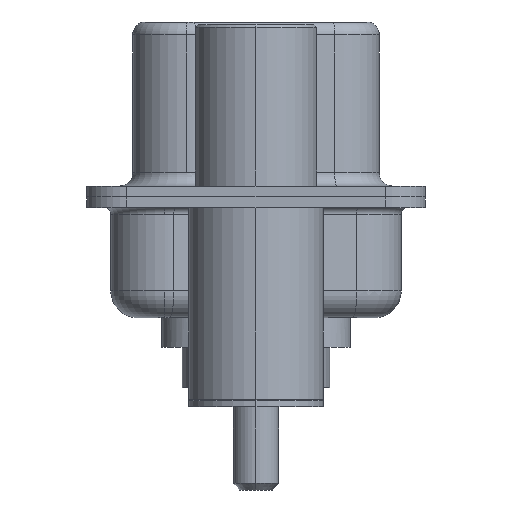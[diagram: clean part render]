
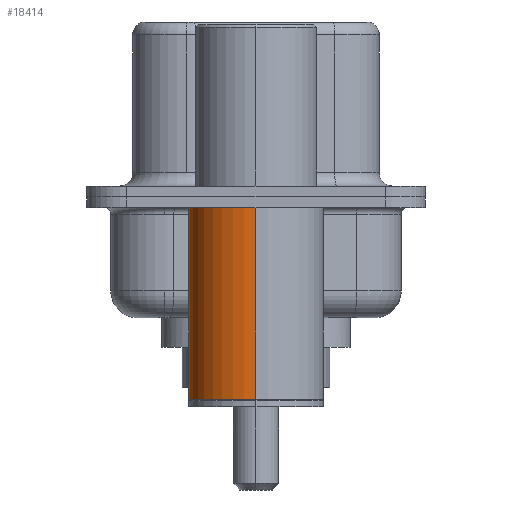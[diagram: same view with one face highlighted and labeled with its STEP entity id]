
A CAD part, left-side view. The second image highlights one B-rep face of the part: STEP entity #18414.
In plain terms, the highlighted cylindrical face has radius 2.5 mm (diameter 5 mm), a partial arc.
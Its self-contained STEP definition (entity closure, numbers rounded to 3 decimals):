
#73 = VERTEX_POINT ( 'NONE', #21918 ) ;
#85 = ORIENTED_EDGE ( 'NONE', *, *, #19931, .T. ) ;
#529 = AXIS2_PLACEMENT_3D ( 'NONE', #9377, #18113, #21693 ) ;
#629 = ORIENTED_EDGE ( 'NONE', *, *, #5912, .F. ) ;
#871 = DIRECTION ( 'NONE',  ( 0., 0., 1. ) ) ;
#2914 = AXIS2_PLACEMENT_3D ( 'NONE', #13565, #18000, #12111 ) ;
#3338 = VERTEX_POINT ( 'NONE', #3787 ) ;
#3787 = CARTESIAN_POINT ( 'NONE',  ( -2.5, 0., -0.4 ) ) ;
#4236 = FACE_OUTER_BOUND ( 'NONE', #6891, .T. ) ;
#5479 = DIRECTION ( 'NONE',  ( 0., 0., 1. ) ) ;
#5726 = CARTESIAN_POINT ( 'NONE',  ( 0., 0., -7.525 ) ) ;
#5912 = EDGE_CURVE ( 'NONE', #7821, #3338, #6349, .T. ) ;
#5987 = CARTESIAN_POINT ( 'NONE',  ( 2.5, 0., -0.4 ) ) ;
#6349 = CIRCLE ( 'NONE', #2914, 2.5 ) ;
#6891 = EDGE_LOOP ( 'NONE', ( #17485, #85, #629, #15341 ) ) ;
#7402 = DIRECTION ( 'NONE',  ( 1., 0., 0. ) ) ;
#7821 = VERTEX_POINT ( 'NONE', #5987 ) ;
#8717 = LINE ( 'NONE', #8789, #17523 ) ;
#8789 = CARTESIAN_POINT ( 'NONE',  ( -2.5, 0., 0.581 ) ) ;
#9377 = CARTESIAN_POINT ( 'NONE',  ( 0., 0., 0.581 ) ) ;
#12032 = LINE ( 'NONE', #21799, #15036 ) ;
#12111 = DIRECTION ( 'NONE',  ( 1., 0., 0. ) ) ;
#13565 = CARTESIAN_POINT ( 'NONE',  ( 0., 0., -0.4 ) ) ;
#15036 = VECTOR ( 'NONE', #871, 1000. ) ;
#15341 = ORIENTED_EDGE ( 'NONE', *, *, #15658, .F. ) ;
#15658 = EDGE_CURVE ( 'NONE', #21307, #7821, #12032, .T. ) ;
#15945 = EDGE_CURVE ( 'NONE', #21307, #73, #21066, .T. ) ;
#17485 = ORIENTED_EDGE ( 'NONE', *, *, #15945, .T. ) ;
#17523 = VECTOR ( 'NONE', #5479, 1000. ) ;
#17882 = DIRECTION ( 'NONE',  ( 0., 0., 1. ) ) ;
#17949 = AXIS2_PLACEMENT_3D ( 'NONE', #5726, #17882, #7402 ) ;
#18000 = DIRECTION ( 'NONE',  ( 0., 0., 1. ) ) ;
#18113 = DIRECTION ( 'NONE',  ( 0., 0., 1. ) ) ;
#18229 = CARTESIAN_POINT ( 'NONE',  ( 2.5, 0., -7.525 ) ) ;
#18414 = ADVANCED_FACE ( 'NONE', ( #4236 ), #21698, .T. ) ;
#19931 = EDGE_CURVE ( 'NONE', #73, #3338, #8717, .T. ) ;
#21066 = CIRCLE ( 'NONE', #17949, 2.5 ) ;
#21307 = VERTEX_POINT ( 'NONE', #18229 ) ;
#21693 = DIRECTION ( 'NONE',  ( 1., 0., 0. ) ) ;
#21698 = CYLINDRICAL_SURFACE ( 'NONE', #529, 2.5 ) ;
#21799 = CARTESIAN_POINT ( 'NONE',  ( 2.5, 0., 0.581 ) ) ;
#21918 = CARTESIAN_POINT ( 'NONE',  ( -2.5, 0., -7.525 ) ) ;
